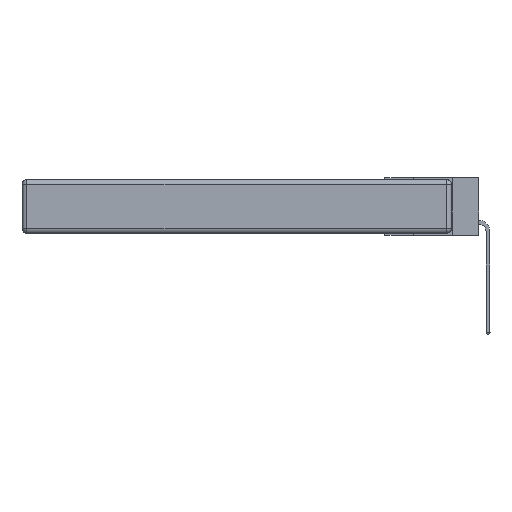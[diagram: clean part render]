
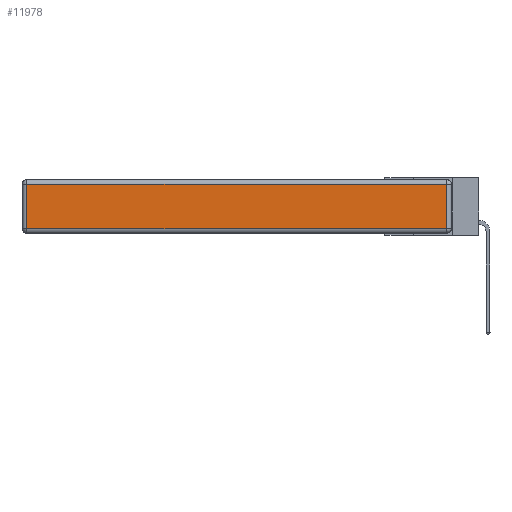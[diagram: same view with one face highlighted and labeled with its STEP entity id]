
A CAD part, left-side view. The second image highlights one B-rep face of the part: STEP entity #11978.
In plain terms, the highlighted planar face has unit normal (-1, 0, 0).
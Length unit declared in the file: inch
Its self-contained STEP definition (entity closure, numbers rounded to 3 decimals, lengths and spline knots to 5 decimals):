
#399 = ORIENTED_EDGE ( 'NONE', *, *, #6096, .T. ) ;
#1190 = CARTESIAN_POINT ( 'NONE',  ( 0., 2.72, -0.313 ) ) ;
#1979 = DIRECTION ( 'NONE',  ( 0., -1., 0. ) ) ;
#2276 = LINE ( 'NONE', #2947, #6012 ) ;
#2735 = DIRECTION ( 'NONE',  ( 0., 0., -1. ) ) ;
#2928 = LINE ( 'NONE', #25742, #5298 ) ;
#2947 = CARTESIAN_POINT ( 'NONE',  ( 0., 2.75, -0.03 ) ) ;
#4222 = CARTESIAN_POINT ( 'NONE',  ( 0., 0., -0.343 ) ) ;
#4322 = PLANE ( 'NONE',  #27736 ) ;
#4546 = VERTEX_POINT ( 'NONE', #6615 ) ;
#5298 = VECTOR ( 'NONE', #24063, 39.37008 ) ;
#5427 = EDGE_CURVE ( 'NONE', #8116, #4546, #20639, .T. ) ;
#6012 = VECTOR ( 'NONE', #11452, 39.37008 ) ;
#6096 = EDGE_CURVE ( 'NONE', #20720, #8116, #6989, .T. ) ;
#6437 = ORIENTED_EDGE ( 'NONE', *, *, #15390, .T. ) ;
#6531 = DIRECTION ( 'NONE',  ( -1., 0., 0. ) ) ;
#6615 = CARTESIAN_POINT ( 'NONE',  ( 0., 0.03, -0.313 ) ) ;
#6989 = LINE ( 'NONE', #26649, #9720 ) ;
#8116 = VERTEX_POINT ( 'NONE', #1190 ) ;
#8513 = CARTESIAN_POINT ( 'NONE',  ( 0., 0., -0.313 ) ) ;
#8865 = DIRECTION ( 'NONE',  ( 0., 0., 1. ) ) ;
#9720 = VECTOR ( 'NONE', #2735, 39.37008 ) ;
#10054 = CARTESIAN_POINT ( 'NONE',  ( 0., 2.72, -0.03 ) ) ;
#10100 = ORIENTED_EDGE ( 'NONE', *, *, #5427, .T. ) ;
#10846 = EDGE_CURVE ( 'NONE', #4546, #14748, #2928, .T. ) ;
#11452 = DIRECTION ( 'NONE',  ( 0., 1., 0. ) ) ;
#11978 = ADVANCED_FACE ( 'NONE', ( #22818 ), #4322, .T. ) ;
#12502 = ORIENTED_EDGE ( 'NONE', *, *, #10846, .T. ) ;
#14158 = CARTESIAN_POINT ( 'NONE',  ( 0., 0.03, -0.03 ) ) ;
#14748 = VERTEX_POINT ( 'NONE', #14158 ) ;
#14997 = EDGE_LOOP ( 'NONE', ( #10100, #12502, #6437, #399 ) ) ;
#15390 = EDGE_CURVE ( 'NONE', #14748, #20720, #2276, .T. ) ;
#20639 = LINE ( 'NONE', #8513, #23964 ) ;
#20720 = VERTEX_POINT ( 'NONE', #10054 ) ;
#22818 = FACE_OUTER_BOUND ( 'NONE', #14997, .T. ) ;
#23964 = VECTOR ( 'NONE', #1979, 39.37008 ) ;
#24063 = DIRECTION ( 'NONE',  ( 0., 0., 1. ) ) ;
#25742 = CARTESIAN_POINT ( 'NONE',  ( 0., 0.03, -0.343 ) ) ;
#26649 = CARTESIAN_POINT ( 'NONE',  ( 0., 2.72, -0.343 ) ) ;
#27736 = AXIS2_PLACEMENT_3D ( 'NONE', #4222, #6531, #8865 ) ;
